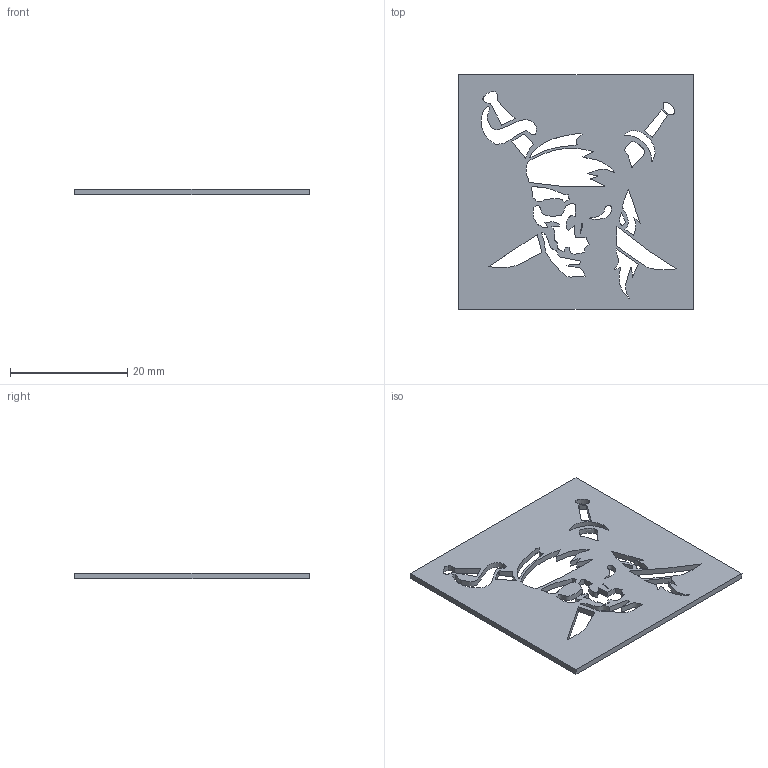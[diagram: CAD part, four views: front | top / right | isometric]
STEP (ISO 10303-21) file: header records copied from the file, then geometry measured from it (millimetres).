
FILE_DESCRIPTION (( 'STEP AP214' ), '1' );
FILE_NAME ('Pirate_Logo.STEP', '2013-09-01T16:54:02', ( 'Asher' ), ( '' ), 'SwSTEP 2.0', 'SolidWorks 2013', '' );
FILE_SCHEMA (( 'AUTOMOTIVE_DESIGN' ));
Length unit declared in the file: millimetre
Products named in the file (1): Pirate_Logo
Bounding box: 40 x 40 x 1 mm (x, y, z)
Volume: 1292.1 mm3; surface area: 3101.6 mm2
Topology: 1 solids, 1 shells, 105 faces, 309 edges, 206 vertices
Faces by surface type: plane 62, bspline 41, cylinder 2
Entity records: 4671 total; most frequent: CARTESIAN_POINT 2042, ORIENTED_EDGE 618, DIRECTION 361, EDGE_CURVE 309, LINE 223, VECTOR 223, VERTEX_POINT 206, EDGE_LOOP 143
